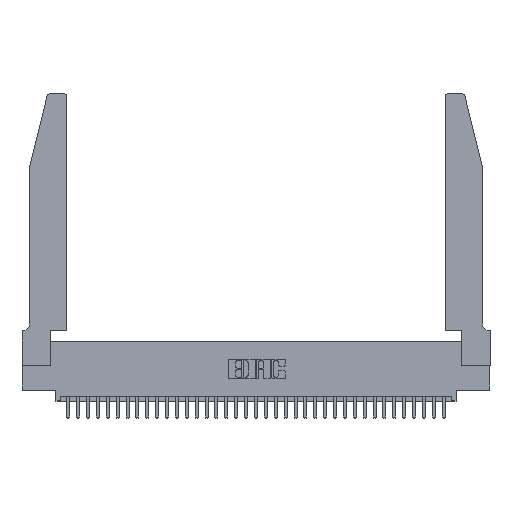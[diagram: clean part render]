
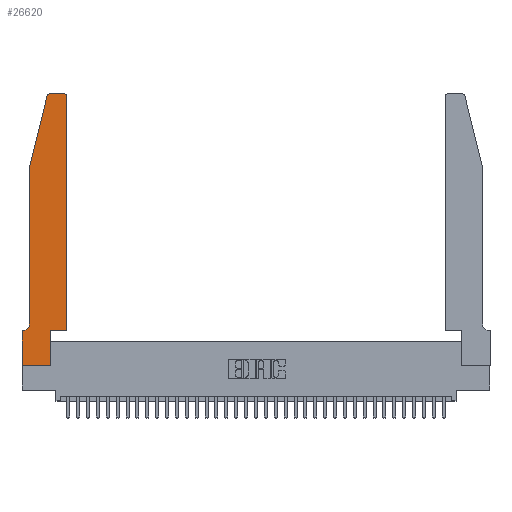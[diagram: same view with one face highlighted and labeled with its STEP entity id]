
A CAD part, top view. The second image highlights one B-rep face of the part: STEP entity #26620.
In plain terms, the highlighted planar face has unit normal (0, 0, 1).
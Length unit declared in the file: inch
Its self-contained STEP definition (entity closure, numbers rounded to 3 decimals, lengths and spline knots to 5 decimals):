
#390 = EDGE_CURVE ( 'NONE', #6583, #7099, #12643, .T. ) ;
#559 = AXIS2_PLACEMENT_3D ( 'NONE', #29591, #33196, #30596 ) ;
#1271 = CARTESIAN_POINT ( 'NONE',  ( 0.4505, 0.35, 0.37 ) ) ;
#2362 = ORIENTED_EDGE ( 'NONE', *, *, #2380, .T. ) ;
#2380 = EDGE_CURVE ( 'NONE', #16168, #32728, #26990, .T. ) ;
#3196 = DIRECTION ( 'NONE',  ( 1., 0., 0. ) ) ;
#3200 = EDGE_CURVE ( 'NONE', #32728, #22252, #11610, .T. ) ;
#3696 = CARTESIAN_POINT ( 'NONE',  ( 0.4205, 2.75, 0.37 ) ) ;
#5525 = CARTESIAN_POINT ( 'NONE',  ( 0.0755, 0.35, 0.37 ) ) ;
#5984 = VECTOR ( 'NONE', #24580, 39.37008 ) ;
#6208 = CARTESIAN_POINT ( 'NONE',  ( 0.2865, 0.35, 0.37 ) ) ;
#6583 = VERTEX_POINT ( 'NONE', #10598 ) ;
#6602 = ORIENTED_EDGE ( 'NONE', *, *, #24394, .T. ) ;
#6625 = EDGE_CURVE ( 'NONE', #7099, #10613, #14812, .T. ) ;
#7099 = VERTEX_POINT ( 'NONE', #33013 ) ;
#7566 = DIRECTION ( 'NONE',  ( -1., 0., 0. ) ) ;
#7727 = CARTESIAN_POINT ( 'NONE',  ( 0.4505, 0.35, 0.37 ) ) ;
#8042 = AXIS2_PLACEMENT_3D ( 'NONE', #24489, #29577, #32503 ) ;
#8513 = ORIENTED_EDGE ( 'NONE', *, *, #6625, .T. ) ;
#8599 = VECTOR ( 'NONE', #23020, 39.37008 ) ;
#9627 = DIRECTION ( 'NONE',  ( 0., -1., 0. ) ) ;
#9954 = EDGE_CURVE ( 'NONE', #11258, #13860, #35027, .T. ) ;
#10348 = ORIENTED_EDGE ( 'NONE', *, *, #11947, .T. ) ;
#10598 = CARTESIAN_POINT ( 'NONE',  ( 0.2865, 0., 0.37 ) ) ;
#10613 = VERTEX_POINT ( 'NONE', #7727 ) ;
#10771 = CARTESIAN_POINT ( 'NONE',  ( 0., 0., 0.37 ) ) ;
#11238 = VERTEX_POINT ( 'NONE', #19566 ) ;
#11258 = VERTEX_POINT ( 'NONE', #29179 ) ;
#11289 = VECTOR ( 'NONE', #15198, 39.37008 ) ;
#11496 = LINE ( 'NONE', #28767, #28112 ) ;
#11610 = LINE ( 'NONE', #30274, #5984 ) ;
#11850 = ORIENTED_EDGE ( 'NONE', *, *, #18415, .T. ) ;
#11947 = EDGE_CURVE ( 'NONE', #17621, #29791, #33171, .T. ) ;
#12375 = DIRECTION ( 'NONE',  ( 0., 0., -1. ) ) ;
#12643 = LINE ( 'NONE', #6208, #34018 ) ;
#12807 = CARTESIAN_POINT ( 'NONE',  ( 0.25487, 2.72718, 0.37 ) ) ;
#13013 = CARTESIAN_POINT ( 'NONE',  ( 0.2605, 2.75, 0.37 ) ) ;
#13860 = VERTEX_POINT ( 'NONE', #3696 ) ;
#13969 = CARTESIAN_POINT ( 'NONE',  ( 0., 0.35, 0.37 ) ) ;
#14812 = LINE ( 'NONE', #16940, #33195 ) ;
#14939 = CARTESIAN_POINT ( 'NONE',  ( 0.4205, 2.72, 0.37 ) ) ;
#15198 = DIRECTION ( 'NONE',  ( -1., 0., 0. ) ) ;
#15660 = EDGE_CURVE ( 'NONE', #22252, #21454, #23459, .T. ) ;
#16010 = ORIENTED_EDGE ( 'NONE', *, *, #9954, .T. ) ;
#16168 = VERTEX_POINT ( 'NONE', #18491 ) ;
#16940 = CARTESIAN_POINT ( 'NONE',  ( 0.4505, 0.35, 0.37 ) ) ;
#17411 = PLANE ( 'NONE',  #559 ) ;
#17621 = VERTEX_POINT ( 'NONE', #29701 ) ;
#18357 = ORIENTED_EDGE ( 'NONE', *, *, #390, .T. ) ;
#18415 = EDGE_CURVE ( 'NONE', #29791, #11238, #11496, .T. ) ;
#18491 = CARTESIAN_POINT ( 'NONE',  ( 0.284, 2.75, 0.37 ) ) ;
#18533 = VECTOR ( 'NONE', #20719, 39.37008 ) ;
#19212 = DIRECTION ( 'NONE',  ( 1., 0., 0. ) ) ;
#19566 = CARTESIAN_POINT ( 'NONE',  ( 0., 0., 0.37 ) ) ;
#19989 = ORIENTED_EDGE ( 'NONE', *, *, #31377, .T. ) ;
#20021 = ORIENTED_EDGE ( 'NONE', *, *, #34827, .T. ) ;
#20431 = VECTOR ( 'NONE', #7566, 39.37008 ) ;
#20571 = ORIENTED_EDGE ( 'NONE', *, *, #15660, .T. ) ;
#20719 = DIRECTION ( 'NONE',  ( 0., 1., 0. ) ) ;
#21190 = ORIENTED_EDGE ( 'NONE', *, *, #33706, .T. ) ;
#21310 = CARTESIAN_POINT ( 'NONE',  ( 0.0755, 0.42, 0.37 ) ) ;
#21454 = VERTEX_POINT ( 'NONE', #21310 ) ;
#22252 = VERTEX_POINT ( 'NONE', #33810 ) ;
#23020 = DIRECTION ( 'NONE',  ( 0., -1., 0. ) ) ;
#23294 = LINE ( 'NONE', #1271, #18533 ) ;
#23374 = DIRECTION ( 'NONE',  ( 0., 0., 1. ) ) ;
#23459 = LINE ( 'NONE', #28480, #8599 ) ;
#23637 = CARTESIAN_POINT ( 'NONE',  ( 0.0055, 0.42, 0.37 ) ) ;
#24220 = VECTOR ( 'NONE', #19212, 39.37008 ) ;
#24394 = EDGE_CURVE ( 'NONE', #10613, #11258, #23294, .T. ) ;
#24489 = CARTESIAN_POINT ( 'NONE',  ( 0.284, 2.72, 0.37 ) ) ;
#24580 = DIRECTION ( 'NONE',  ( -0.239, -0.971, 0. ) ) ;
#25735 = DIRECTION ( 'NONE',  ( 0., 1., 0. ) ) ;
#26184 = DIRECTION ( 'NONE',  ( 1., 0., 0. ) ) ;
#26620 = ADVANCED_FACE ( 'NONE', ( #33610 ), #17411, .T. ) ;
#26990 = CIRCLE ( 'NONE', #8042, 0.03 ) ;
#27877 = AXIS2_PLACEMENT_3D ( 'NONE', #23637, #12375, #29332 ) ;
#28112 = VECTOR ( 'NONE', #9627, 39.37008 ) ;
#28480 = CARTESIAN_POINT ( 'NONE',  ( 0.0755, 2., 0.37 ) ) ;
#28767 = CARTESIAN_POINT ( 'NONE',  ( 0., 0., 0.37 ) ) ;
#28897 = AXIS2_PLACEMENT_3D ( 'NONE', #14939, #23374, #26184 ) ;
#29179 = CARTESIAN_POINT ( 'NONE',  ( 0.4505, 2.72, 0.37 ) ) ;
#29332 = DIRECTION ( 'NONE',  ( -1., 0., 0. ) ) ;
#29577 = DIRECTION ( 'NONE',  ( 0., 0., 1. ) ) ;
#29591 = CARTESIAN_POINT ( 'NONE',  ( 0., 0.35, 0.37 ) ) ;
#29701 = CARTESIAN_POINT ( 'NONE',  ( 0.0055, 0.35, 0.37 ) ) ;
#29791 = VERTEX_POINT ( 'NONE', #13969 ) ;
#30274 = CARTESIAN_POINT ( 'NONE',  ( 0.0755, 2., 0.37 ) ) ;
#30596 = DIRECTION ( 'NONE',  ( 1., 0., 0. ) ) ;
#31153 = ORIENTED_EDGE ( 'NONE', *, *, #3200, .T. ) ;
#31377 = EDGE_CURVE ( 'NONE', #13860, #16168, #35281, .T. ) ;
#31589 = LINE ( 'NONE', #10771, #24220 ) ;
#32503 = DIRECTION ( 'NONE',  ( 1., 0., 0. ) ) ;
#32728 = VERTEX_POINT ( 'NONE', #12807 ) ;
#33013 = CARTESIAN_POINT ( 'NONE',  ( 0.2865, 0.35, 0.37 ) ) ;
#33171 = LINE ( 'NONE', #5525, #11289 ) ;
#33195 = VECTOR ( 'NONE', #3196, 39.37008 ) ;
#33196 = DIRECTION ( 'NONE',  ( 0., 0., 1. ) ) ;
#33610 = FACE_OUTER_BOUND ( 'NONE', #34176, .T. ) ;
#33706 = EDGE_CURVE ( 'NONE', #11238, #6583, #31589, .T. ) ;
#33810 = CARTESIAN_POINT ( 'NONE',  ( 0.0755, 2., 0.37 ) ) ;
#34018 = VECTOR ( 'NONE', #25735, 39.37008 ) ;
#34176 = EDGE_LOOP ( 'NONE', ( #19989, #2362, #31153, #20571, #20021, #10348, #11850, #21190, #18357, #8513, #6602, #16010 ) ) ;
#34827 = EDGE_CURVE ( 'NONE', #21454, #17621, #35900, .T. ) ;
#35027 = CIRCLE ( 'NONE', #28897, 0.03 ) ;
#35281 = LINE ( 'NONE', #13013, #20431 ) ;
#35900 = CIRCLE ( 'NONE', #27877, 0.07 ) ;
